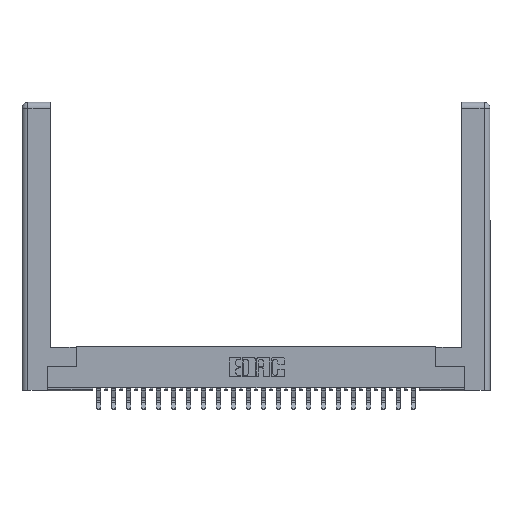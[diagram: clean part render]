
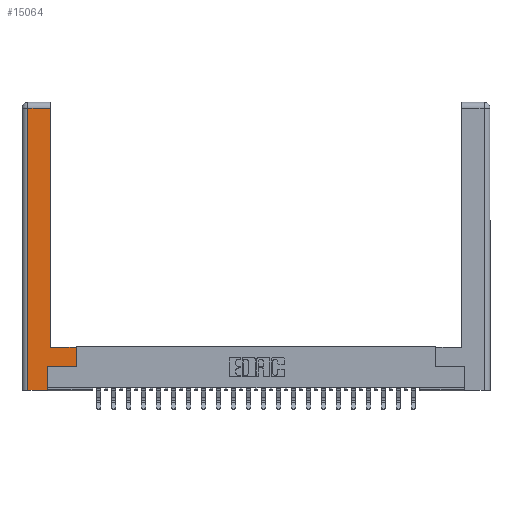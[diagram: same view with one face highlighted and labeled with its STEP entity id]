
A CAD part, top view. The second image highlights one B-rep face of the part: STEP entity #15064.
In plain terms, the highlighted planar face has unit normal (0, 0, 1).
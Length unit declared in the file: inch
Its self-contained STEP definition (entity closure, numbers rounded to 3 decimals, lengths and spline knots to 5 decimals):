
#154 = VECTOR ( 'NONE', #28971, 39.37008 ) ;
#439 = CARTESIAN_POINT ( 'NONE',  ( 0.295, 0.45, 0. ) ) ;
#1012 = EDGE_CURVE ( 'NONE', #3479, #18481, #21948, .T. ) ;
#1175 = ORIENTED_EDGE ( 'NONE', *, *, #24995, .T. ) ;
#1190 = LINE ( 'NONE', #24480, #154 ) ;
#1746 = CARTESIAN_POINT ( 'NONE',  ( 0.0615, 2.94, 0. ) ) ;
#2107 = DIRECTION ( 'NONE',  ( 1., 0., 0. ) ) ;
#2788 = LINE ( 'NONE', #19699, #9147 ) ;
#3344 = VECTOR ( 'NONE', #18265, 39.37008 ) ;
#3479 = VERTEX_POINT ( 'NONE', #7273 ) ;
#4154 = VECTOR ( 'NONE', #23358, 39.37008 ) ;
#4368 = DIRECTION ( 'NONE',  ( 0., 1., 0. ) ) ;
#4449 = VECTOR ( 'NONE', #2107, 39.37008 ) ;
#5184 = EDGE_CURVE ( 'NONE', #11612, #21641, #13877, .T. ) ;
#6077 = ORIENTED_EDGE ( 'NONE', *, *, #11297, .T. ) ;
#6210 = AXIS2_PLACEMENT_3D ( 'NONE', #7221, #9478, #7319 ) ;
#6254 = LINE ( 'NONE', #18422, #4154 ) ;
#6625 = CARTESIAN_POINT ( 'NONE',  ( 0.565, 0.245, 0. ) ) ;
#7024 = PLANE ( 'NONE',  #6210 ) ;
#7221 = CARTESIAN_POINT ( 'NONE',  ( 0., 0., 0. ) ) ;
#7273 = CARTESIAN_POINT ( 'NONE',  ( 0.565, 0.45, 0. ) ) ;
#7319 = DIRECTION ( 'NONE',  ( -1., 0., 0. ) ) ;
#7405 = LINE ( 'NONE', #1746, #13686 ) ;
#8180 = ORIENTED_EDGE ( 'NONE', *, *, #21565, .T. ) ;
#9096 = VERTEX_POINT ( 'NONE', #11323 ) ;
#9147 = VECTOR ( 'NONE', #21987, 39.37008 ) ;
#9478 = DIRECTION ( 'NONE',  ( 0., 0., -1. ) ) ;
#10349 = FACE_OUTER_BOUND ( 'NONE', #24278, .T. ) ;
#10415 = LINE ( 'NONE', #6625, #4449 ) ;
#11297 = EDGE_CURVE ( 'NONE', #9096, #12680, #7405, .T. ) ;
#11323 = CARTESIAN_POINT ( 'NONE',  ( 0.295, 2.94, 0. ) ) ;
#11612 = VERTEX_POINT ( 'NONE', #19795 ) ;
#12255 = VERTEX_POINT ( 'NONE', #24965 ) ;
#12680 = VERTEX_POINT ( 'NONE', #18139 ) ;
#13681 = CARTESIAN_POINT ( 'NONE',  ( 0.295, 0.45, 0. ) ) ;
#13686 = VECTOR ( 'NONE', #22027, 39.37008 ) ;
#13877 = LINE ( 'NONE', #25065, #3344 ) ;
#14393 = VECTOR ( 'NONE', #4368, 39.37008 ) ;
#15064 = ADVANCED_FACE ( 'NONE', ( #10349 ), #7024, .F. ) ;
#16161 = EDGE_CURVE ( 'NONE', #12680, #12255, #6254, .T. ) ;
#17146 = ORIENTED_EDGE ( 'NONE', *, *, #5184, .T. ) ;
#18032 = CARTESIAN_POINT ( 'NONE',  ( 0.565, 0.45, 0. ) ) ;
#18139 = CARTESIAN_POINT ( 'NONE',  ( 0.0615, 2.94, 0. ) ) ;
#18265 = DIRECTION ( 'NONE',  ( 0., 1., 0. ) ) ;
#18422 = CARTESIAN_POINT ( 'NONE',  ( 0.0615, 0., 0. ) ) ;
#18481 = VERTEX_POINT ( 'NONE', #13681 ) ;
#19699 = CARTESIAN_POINT ( 'NONE',  ( 0.265, 0., 0. ) ) ;
#19795 = CARTESIAN_POINT ( 'NONE',  ( 0.265, 0., 0. ) ) ;
#19850 = EDGE_CURVE ( 'NONE', #12255, #11612, #2788, .T. ) ;
#21565 = EDGE_CURVE ( 'NONE', #21641, #24254, #10415, .T. ) ;
#21641 = VERTEX_POINT ( 'NONE', #27084 ) ;
#21948 = LINE ( 'NONE', #439, #26514 ) ;
#21987 = DIRECTION ( 'NONE',  ( 1., 0., 0. ) ) ;
#22027 = DIRECTION ( 'NONE',  ( -1., 0., 0. ) ) ;
#23358 = DIRECTION ( 'NONE',  ( 0., -1., 0. ) ) ;
#24254 = VERTEX_POINT ( 'NONE', #25237 ) ;
#24278 = EDGE_LOOP ( 'NONE', ( #1175, #6077, #26029, #26468, #17146, #8180, #28591, #26269 ) ) ;
#24480 = CARTESIAN_POINT ( 'NONE',  ( 0.295, 3., 0. ) ) ;
#24965 = CARTESIAN_POINT ( 'NONE',  ( 0.0615, 0., 0. ) ) ;
#24995 = EDGE_CURVE ( 'NONE', #18481, #9096, #1190, .T. ) ;
#25065 = CARTESIAN_POINT ( 'NONE',  ( 0.265, 0.245, 0. ) ) ;
#25237 = CARTESIAN_POINT ( 'NONE',  ( 0.565, 0.245, 0. ) ) ;
#25307 = DIRECTION ( 'NONE',  ( -1., 0., 0. ) ) ;
#26029 = ORIENTED_EDGE ( 'NONE', *, *, #16161, .T. ) ;
#26269 = ORIENTED_EDGE ( 'NONE', *, *, #1012, .T. ) ;
#26372 = LINE ( 'NONE', #18032, #14393 ) ;
#26468 = ORIENTED_EDGE ( 'NONE', *, *, #19850, .T. ) ;
#26514 = VECTOR ( 'NONE', #25307, 39.37008 ) ;
#27084 = CARTESIAN_POINT ( 'NONE',  ( 0.265, 0.245, 0. ) ) ;
#27799 = EDGE_CURVE ( 'NONE', #24254, #3479, #26372, .T. ) ;
#28591 = ORIENTED_EDGE ( 'NONE', *, *, #27799, .T. ) ;
#28971 = DIRECTION ( 'NONE',  ( 0., 1., 0. ) ) ;
